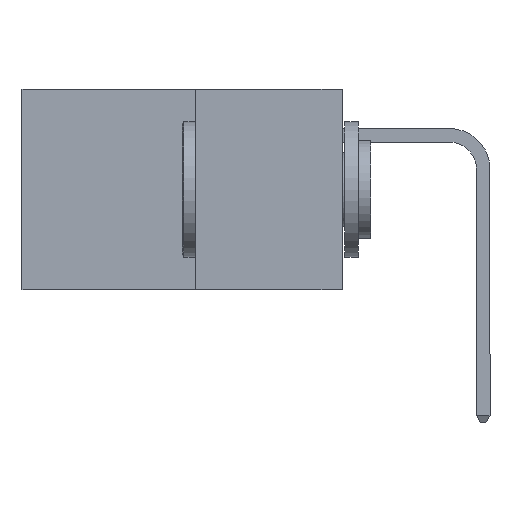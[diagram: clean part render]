
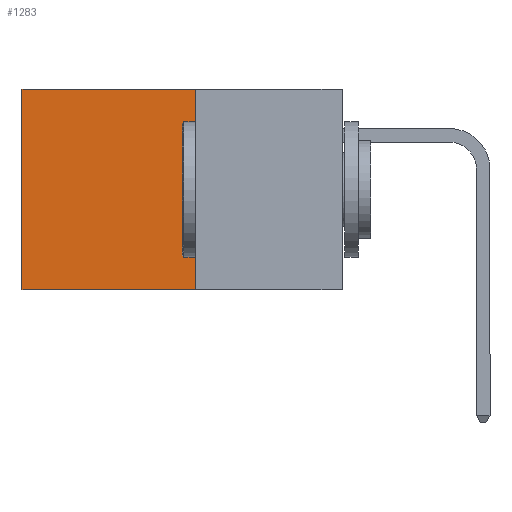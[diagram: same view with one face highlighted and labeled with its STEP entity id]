
A CAD part, left-side view. The second image highlights one B-rep face of the part: STEP entity #1283.
In plain terms, the highlighted planar face has unit normal (-1, 0, 0).
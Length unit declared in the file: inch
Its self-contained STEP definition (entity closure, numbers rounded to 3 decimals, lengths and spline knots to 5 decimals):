
#426 = EDGE_CURVE ( 'NONE', #7667, #1644, #9935, .T. ) ;
#433 = PLANE ( 'NONE',  #7934 ) ;
#902 = ORIENTED_EDGE ( 'NONE', *, *, #8896, .F. ) ;
#1283 = ADVANCED_FACE ( 'NONE', ( #3266 ), #433, .F. ) ;
#1644 = VERTEX_POINT ( 'NONE', #3376 ) ;
#1811 = DIRECTION ( 'NONE',  ( 0., 0., -1. ) ) ;
#2188 = CARTESIAN_POINT ( 'NONE',  ( 0.277, 0.59, -0.37 ) ) ;
#2265 = CARTESIAN_POINT ( 'NONE',  ( 0.277, 0.27, -0.37 ) ) ;
#2741 = VECTOR ( 'NONE', #10919, 39.37008 ) ;
#3250 = ORIENTED_EDGE ( 'NONE', *, *, #426, .T. ) ;
#3266 = FACE_OUTER_BOUND ( 'NONE', #6858, .T. ) ;
#3376 = CARTESIAN_POINT ( 'NONE',  ( 0.277, 0.59, 0. ) ) ;
#3655 = VERTEX_POINT ( 'NONE', #2265 ) ;
#4147 = LINE ( 'NONE', #8848, #10978 ) ;
#4679 = EDGE_CURVE ( 'NONE', #3655, #5291, #4147, .T. ) ;
#5291 = VERTEX_POINT ( 'NONE', #9976 ) ;
#5329 = CARTESIAN_POINT ( 'NONE',  ( 0.277, 0.27, 0. ) ) ;
#5450 = VECTOR ( 'NONE', #8326, 39.37008 ) ;
#5593 = LINE ( 'NONE', #7037, #7869 ) ;
#6858 = EDGE_LOOP ( 'NONE', ( #7573, #9889, #902, #3250 ) ) ;
#7037 = CARTESIAN_POINT ( 'NONE',  ( 0.277, 0.27, -0.37 ) ) ;
#7573 = ORIENTED_EDGE ( 'NONE', *, *, #8675, .T. ) ;
#7667 = VERTEX_POINT ( 'NONE', #5329 ) ;
#7869 = VECTOR ( 'NONE', #1811, 39.37008 ) ;
#7934 = AXIS2_PLACEMENT_3D ( 'NONE', #11104, #8932, #9797 ) ;
#8326 = DIRECTION ( 'NONE',  ( 0., 0., -1. ) ) ;
#8675 = EDGE_CURVE ( 'NONE', #1644, #5291, #10062, .T. ) ;
#8848 = CARTESIAN_POINT ( 'NONE',  ( 0.277, 0.27, -0.37 ) ) ;
#8896 = EDGE_CURVE ( 'NONE', #7667, #3655, #5593, .T. ) ;
#8932 = DIRECTION ( 'NONE',  ( 1., 0., 0. ) ) ;
#9518 = CARTESIAN_POINT ( 'NONE',  ( 0.277, 0.27, 0. ) ) ;
#9797 = DIRECTION ( 'NONE',  ( 0., 0., -1. ) ) ;
#9831 = DIRECTION ( 'NONE',  ( 0., 1., 0. ) ) ;
#9889 = ORIENTED_EDGE ( 'NONE', *, *, #4679, .F. ) ;
#9935 = LINE ( 'NONE', #9518, #2741 ) ;
#9976 = CARTESIAN_POINT ( 'NONE',  ( 0.277, 0.59, -0.37 ) ) ;
#10062 = LINE ( 'NONE', #2188, #5450 ) ;
#10919 = DIRECTION ( 'NONE',  ( 0., 1., 0. ) ) ;
#10978 = VECTOR ( 'NONE', #9831, 39.37008 ) ;
#11104 = CARTESIAN_POINT ( 'NONE',  ( 0.277, 0.27, -0.37 ) ) ;
